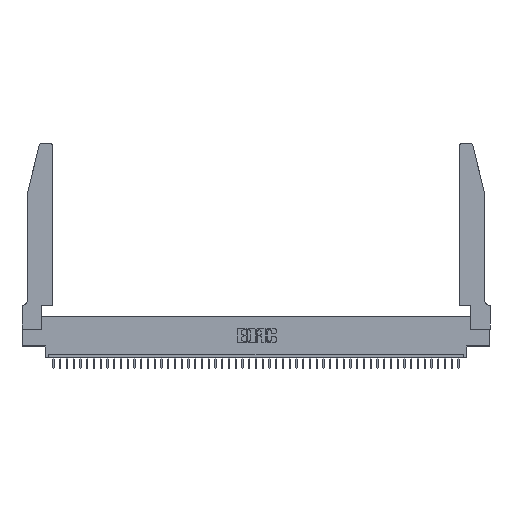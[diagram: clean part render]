
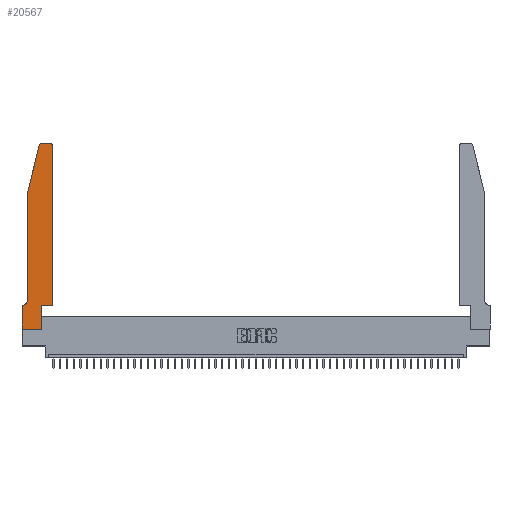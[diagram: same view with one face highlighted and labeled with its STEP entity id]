
A CAD part, top view. The second image highlights one B-rep face of the part: STEP entity #20567.
In plain terms, the highlighted planar face has unit normal (0, 0, 1).
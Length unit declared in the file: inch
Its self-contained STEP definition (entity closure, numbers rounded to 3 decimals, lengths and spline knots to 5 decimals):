
#404 = VERTEX_POINT ( 'NONE', #5575 ) ;
#1081 = CARTESIAN_POINT ( 'NONE',  ( 0.0055, 0.35, 0.37 ) ) ;
#1163 = AXIS2_PLACEMENT_3D ( 'NONE', #39693, #9483, #35634 ) ;
#1620 = ORIENTED_EDGE ( 'NONE', *, *, #34897, .T. ) ;
#1625 = EDGE_CURVE ( 'NONE', #28419, #3823, #22523, .T. ) ;
#1648 = EDGE_CURVE ( 'NONE', #33592, #43917, #32537, .T. ) ;
#1906 = CARTESIAN_POINT ( 'NONE',  ( 0., 0., 0.37 ) ) ;
#1921 = VERTEX_POINT ( 'NONE', #42820 ) ;
#1951 = CARTESIAN_POINT ( 'NONE',  ( 0.0055, 0.42, 0.37 ) ) ;
#2144 = VECTOR ( 'NONE', #14307, 39.37008 ) ;
#2472 = AXIS2_PLACEMENT_3D ( 'NONE', #40904, #44915, #14790 ) ;
#2713 = DIRECTION ( 'NONE',  ( 0., 0., 1. ) ) ;
#3526 = LINE ( 'NONE', #1906, #18671 ) ;
#3823 = VERTEX_POINT ( 'NONE', #17598 ) ;
#5265 = VECTOR ( 'NONE', #19047, 39.37008 ) ;
#5575 = CARTESIAN_POINT ( 'NONE',  ( 0., 0.35, 0.37 ) ) ;
#5695 = VECTOR ( 'NONE', #13364, 39.37008 ) ;
#5977 = DIRECTION ( 'NONE',  ( 0., -1., 0. ) ) ;
#6277 = AXIS2_PLACEMENT_3D ( 'NONE', #21148, #2713, #29014 ) ;
#6416 = ORIENTED_EDGE ( 'NONE', *, *, #14465, .T. ) ;
#9483 = DIRECTION ( 'NONE',  ( 0., 0., 1. ) ) ;
#10425 = VERTEX_POINT ( 'NONE', #28008 ) ;
#10839 = LINE ( 'NONE', #31631, #47621 ) ;
#11705 = CARTESIAN_POINT ( 'NONE',  ( 0.0755, 0.35, 0.37 ) ) ;
#11753 = VECTOR ( 'NONE', #16224, 39.37008 ) ;
#13003 = DIRECTION ( 'NONE',  ( 1., 0., 0. ) ) ;
#13364 = DIRECTION ( 'NONE',  ( 0., 1., 0. ) ) ;
#13643 = VERTEX_POINT ( 'NONE', #47498 ) ;
#14307 = DIRECTION ( 'NONE',  ( 0., -1., 0. ) ) ;
#14465 = EDGE_CURVE ( 'NONE', #13643, #14516, #16593, .T. ) ;
#14516 = VERTEX_POINT ( 'NONE', #45554 ) ;
#14790 = DIRECTION ( 'NONE',  ( 1., 0., 0. ) ) ;
#15224 = LINE ( 'NONE', #11705, #5265 ) ;
#16224 = DIRECTION ( 'NONE',  ( 1., 0., 0. ) ) ;
#16593 = LINE ( 'NONE', #26209, #32411 ) ;
#16631 = ORIENTED_EDGE ( 'NONE', *, *, #31124, .T. ) ;
#17171 = AXIS2_PLACEMENT_3D ( 'NONE', #1951, #39040, #20553 ) ;
#17598 = CARTESIAN_POINT ( 'NONE',  ( 0.4205, 2.75, 0.37 ) ) ;
#18269 = EDGE_CURVE ( 'NONE', #37621, #1921, #10839, .T. ) ;
#18671 = VECTOR ( 'NONE', #5977, 39.37008 ) ;
#18693 = ORIENTED_EDGE ( 'NONE', *, *, #36415, .T. ) ;
#19047 = DIRECTION ( 'NONE',  ( -1., 0., 0. ) ) ;
#19722 = VECTOR ( 'NONE', #26356, 39.37008 ) ;
#19854 = ORIENTED_EDGE ( 'NONE', *, *, #32176, .T. ) ;
#20150 = ORIENTED_EDGE ( 'NONE', *, *, #31385, .T. ) ;
#20553 = DIRECTION ( 'NONE',  ( -1., 0., 0. ) ) ;
#20567 = ADVANCED_FACE ( 'NONE', ( #24568 ), #38974, .T. ) ;
#21029 = CARTESIAN_POINT ( 'NONE',  ( 0.2865, 0.35, 0.37 ) ) ;
#21107 = EDGE_CURVE ( 'NONE', #404, #43958, #3526, .T. ) ;
#21116 = LINE ( 'NONE', #38444, #11753 ) ;
#21148 = CARTESIAN_POINT ( 'NONE',  ( 0., 0.35, 0.37 ) ) ;
#21909 = CARTESIAN_POINT ( 'NONE',  ( 0.2865, 0.35, 0.37 ) ) ;
#22523 = CIRCLE ( 'NONE', #1163, 0.03 ) ;
#22575 = CARTESIAN_POINT ( 'NONE',  ( 0.2605, 2.75, 0.37 ) ) ;
#23369 = DIRECTION ( 'NONE',  ( -0.239, -0.971, 0. ) ) ;
#24568 = FACE_OUTER_BOUND ( 'NONE', #36052, .T. ) ;
#25597 = VECTOR ( 'NONE', #47536, 39.37008 ) ;
#25992 = CARTESIAN_POINT ( 'NONE',  ( 0.0755, 0.42, 0.37 ) ) ;
#26209 = CARTESIAN_POINT ( 'NONE',  ( 0.0755, 2., 0.37 ) ) ;
#26356 = DIRECTION ( 'NONE',  ( -1., 0., 0. ) ) ;
#27076 = VERTEX_POINT ( 'NONE', #27733 ) ;
#27430 = ORIENTED_EDGE ( 'NONE', *, *, #1648, .T. ) ;
#27733 = CARTESIAN_POINT ( 'NONE',  ( 0.2865, 0., 0.37 ) ) ;
#27915 = CARTESIAN_POINT ( 'NONE',  ( 0., 0., 0.37 ) ) ;
#28008 = CARTESIAN_POINT ( 'NONE',  ( 0.284, 2.75, 0.37 ) ) ;
#28419 = VERTEX_POINT ( 'NONE', #43786 ) ;
#28492 = ORIENTED_EDGE ( 'NONE', *, *, #18269, .T. ) ;
#29014 = DIRECTION ( 'NONE',  ( 1., 0., 0. ) ) ;
#29469 = ORIENTED_EDGE ( 'NONE', *, *, #1625, .T. ) ;
#30140 = CIRCLE ( 'NONE', #2472, 0.03 ) ;
#31124 = EDGE_CURVE ( 'NONE', #3823, #10425, #40250, .T. ) ;
#31385 = EDGE_CURVE ( 'NONE', #27076, #37621, #36700, .T. ) ;
#31631 = CARTESIAN_POINT ( 'NONE',  ( 0.4505, 0.35, 0.37 ) ) ;
#32176 = EDGE_CURVE ( 'NONE', #14516, #33592, #48238, .T. ) ;
#32411 = VECTOR ( 'NONE', #23369, 39.37008 ) ;
#32537 = CIRCLE ( 'NONE', #17171, 0.07 ) ;
#33592 = VERTEX_POINT ( 'NONE', #25992 ) ;
#34275 = ORIENTED_EDGE ( 'NONE', *, *, #37437, .T. ) ;
#34897 = EDGE_CURVE ( 'NONE', #43958, #27076, #21116, .T. ) ;
#35634 = DIRECTION ( 'NONE',  ( 1., 0., 0. ) ) ;
#36052 = EDGE_LOOP ( 'NONE', ( #16631, #48173, #6416, #19854, #27430, #18693, #44924, #1620, #20150, #28492, #34275, #29469 ) ) ;
#36161 = LINE ( 'NONE', #40242, #25597 ) ;
#36415 = EDGE_CURVE ( 'NONE', #43917, #404, #15224, .T. ) ;
#36700 = LINE ( 'NONE', #21029, #5695 ) ;
#37437 = EDGE_CURVE ( 'NONE', #1921, #28419, #36161, .T. ) ;
#37621 = VERTEX_POINT ( 'NONE', #21909 ) ;
#38444 = CARTESIAN_POINT ( 'NONE',  ( 0., 0., 0.37 ) ) ;
#38801 = EDGE_CURVE ( 'NONE', #10425, #13643, #30140, .T. ) ;
#38974 = PLANE ( 'NONE',  #6277 ) ;
#39040 = DIRECTION ( 'NONE',  ( 0., 0., -1. ) ) ;
#39693 = CARTESIAN_POINT ( 'NONE',  ( 0.4205, 2.72, 0.37 ) ) ;
#40242 = CARTESIAN_POINT ( 'NONE',  ( 0.4505, 0.35, 0.37 ) ) ;
#40250 = LINE ( 'NONE', #22575, #19722 ) ;
#40904 = CARTESIAN_POINT ( 'NONE',  ( 0.284, 2.72, 0.37 ) ) ;
#42820 = CARTESIAN_POINT ( 'NONE',  ( 0.4505, 0.35, 0.37 ) ) ;
#43786 = CARTESIAN_POINT ( 'NONE',  ( 0.4505, 2.72, 0.37 ) ) ;
#43917 = VERTEX_POINT ( 'NONE', #1081 ) ;
#43958 = VERTEX_POINT ( 'NONE', #27915 ) ;
#44915 = DIRECTION ( 'NONE',  ( 0., 0., 1. ) ) ;
#44924 = ORIENTED_EDGE ( 'NONE', *, *, #21107, .T. ) ;
#45554 = CARTESIAN_POINT ( 'NONE',  ( 0.0755, 2., 0.37 ) ) ;
#47498 = CARTESIAN_POINT ( 'NONE',  ( 0.25487, 2.72718, 0.37 ) ) ;
#47536 = DIRECTION ( 'NONE',  ( 0., 1., 0. ) ) ;
#47621 = VECTOR ( 'NONE', #13003, 39.37008 ) ;
#48057 = CARTESIAN_POINT ( 'NONE',  ( 0.0755, 2., 0.37 ) ) ;
#48173 = ORIENTED_EDGE ( 'NONE', *, *, #38801, .T. ) ;
#48238 = LINE ( 'NONE', #48057, #2144 ) ;
